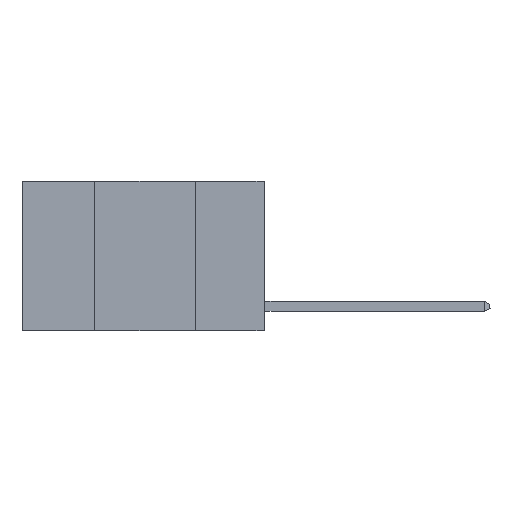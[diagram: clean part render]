
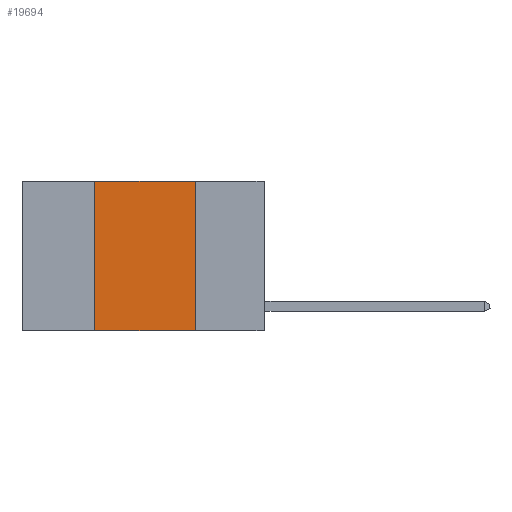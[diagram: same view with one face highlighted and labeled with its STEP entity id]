
A CAD part, left-side view. The second image highlights one B-rep face of the part: STEP entity #19694.
In plain terms, the highlighted planar face has unit normal (-1, 0, 0).
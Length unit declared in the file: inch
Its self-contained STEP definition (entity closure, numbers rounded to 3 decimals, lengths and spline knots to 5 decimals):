
#100 = ORIENTED_EDGE ( 'NONE', *, *, #15786, .T. ) ;
#1165 = DIRECTION ( 'NONE',  ( 0., 0., 1. ) ) ;
#2051 = VECTOR ( 'NONE', #16002, 39.37008 ) ;
#2508 = VECTOR ( 'NONE', #1165, 39.37008 ) ;
#3016 = ORIENTED_EDGE ( 'NONE', *, *, #9154, .F. ) ;
#3119 = PLANE ( 'NONE',  #11655 ) ;
#3304 = CARTESIAN_POINT ( 'NONE',  ( 0., 0.42, 0. ) ) ;
#4758 = VERTEX_POINT ( 'NONE', #6585 ) ;
#4892 = CARTESIAN_POINT ( 'NONE',  ( 0., 0.17, -0.37 ) ) ;
#5595 = EDGE_CURVE ( 'NONE', #4758, #9637, #19302, .T. ) ;
#6449 = LINE ( 'NONE', #17511, #11306 ) ;
#6585 = CARTESIAN_POINT ( 'NONE',  ( 0., 0.17, 0. ) ) ;
#6834 = VERTEX_POINT ( 'NONE', #3304 ) ;
#8221 = CARTESIAN_POINT ( 'NONE',  ( 0., 0.17, 0. ) ) ;
#8822 = VECTOR ( 'NONE', #12682, 39.37008 ) ;
#9136 = LINE ( 'NONE', #20638, #2508 ) ;
#9154 = EDGE_CURVE ( 'NONE', #18369, #6834, #9136, .T. ) ;
#9475 = ORIENTED_EDGE ( 'NONE', *, *, #19047, .F. ) ;
#9637 = VERTEX_POINT ( 'NONE', #4892 ) ;
#9694 = DIRECTION ( 'NONE',  ( 0., -1., 0. ) ) ;
#10870 = FACE_OUTER_BOUND ( 'NONE', #13351, .T. ) ;
#11306 = VECTOR ( 'NONE', #9694, 39.37008 ) ;
#11655 = AXIS2_PLACEMENT_3D ( 'NONE', #12563, #14241, #15825 ) ;
#12563 = CARTESIAN_POINT ( 'NONE',  ( 0., 0.6, 0. ) ) ;
#12682 = DIRECTION ( 'NONE',  ( 0., -1., 0. ) ) ;
#13351 = EDGE_LOOP ( 'NONE', ( #15996, #9475, #3016, #100 ) ) ;
#14241 = DIRECTION ( 'NONE',  ( 1., 0., 0. ) ) ;
#15786 = EDGE_CURVE ( 'NONE', #18369, #9637, #17763, .T. ) ;
#15825 = DIRECTION ( 'NONE',  ( 0., 0., -1. ) ) ;
#15996 = ORIENTED_EDGE ( 'NONE', *, *, #5595, .F. ) ;
#16002 = DIRECTION ( 'NONE',  ( 0., 0., -1. ) ) ;
#16057 = CARTESIAN_POINT ( 'NONE',  ( 0., 0.6, -0.37 ) ) ;
#17511 = CARTESIAN_POINT ( 'NONE',  ( 0., 0.6, 0. ) ) ;
#17763 = LINE ( 'NONE', #16057, #8822 ) ;
#18369 = VERTEX_POINT ( 'NONE', #19709 ) ;
#19047 = EDGE_CURVE ( 'NONE', #6834, #4758, #6449, .T. ) ;
#19302 = LINE ( 'NONE', #8221, #2051 ) ;
#19694 = ADVANCED_FACE ( 'NONE', ( #10870 ), #3119, .F. ) ;
#19709 = CARTESIAN_POINT ( 'NONE',  ( 0., 0.42, -0.37 ) ) ;
#20638 = CARTESIAN_POINT ( 'NONE',  ( 0., 0.42, 0. ) ) ;
